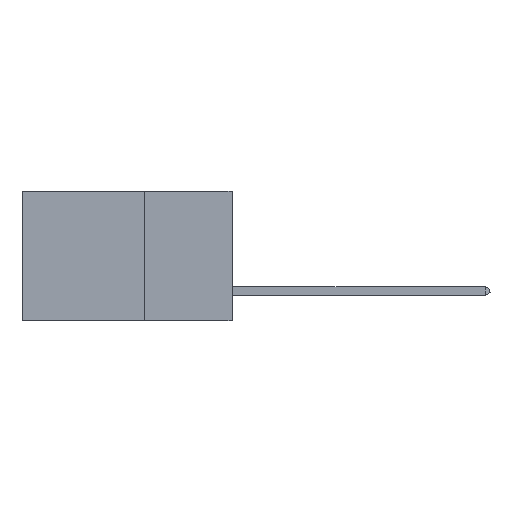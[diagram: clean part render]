
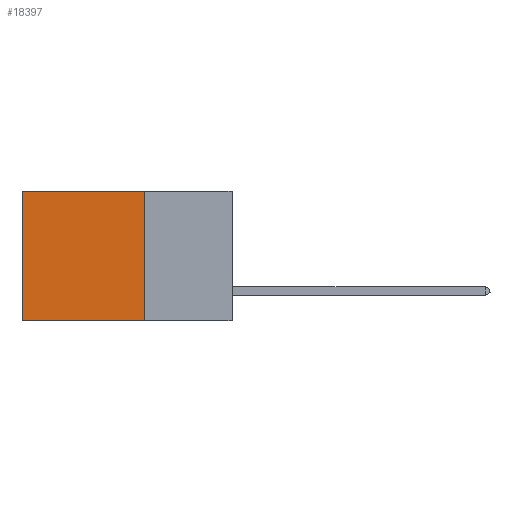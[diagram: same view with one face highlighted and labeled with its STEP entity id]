
A CAD part, left-side view. The second image highlights one B-rep face of the part: STEP entity #18397.
In plain terms, the highlighted planar face has unit normal (-1, 0, 0).
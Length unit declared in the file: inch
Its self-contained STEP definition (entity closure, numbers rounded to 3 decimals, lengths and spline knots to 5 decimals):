
#1252 = VECTOR ( 'NONE', #1528, 39.37008 ) ;
#1479 = VERTEX_POINT ( 'NONE', #2899 ) ;
#1528 = DIRECTION ( 'NONE',  ( 0., 0., -1. ) ) ;
#1542 = VERTEX_POINT ( 'NONE', #2821 ) ;
#2821 = CARTESIAN_POINT ( 'NONE',  ( 0.2875, 0.6, 0. ) ) ;
#2899 = CARTESIAN_POINT ( 'NONE',  ( 0.2875, 0.25, 0. ) ) ;
#3000 = EDGE_CURVE ( 'NONE', #1479, #17118, #3886, .T. ) ;
#3084 = EDGE_CURVE ( 'NONE', #1479, #1542, #9655, .T. ) ;
#3738 = ORIENTED_EDGE ( 'NONE', *, *, #3084, .T. ) ;
#3886 = LINE ( 'NONE', #14391, #18161 ) ;
#4565 = CARTESIAN_POINT ( 'NONE',  ( 0.2875, 0.25, -0.37 ) ) ;
#4890 = CARTESIAN_POINT ( 'NONE',  ( 0.2875, 0.25, -0.37 ) ) ;
#5632 = VECTOR ( 'NONE', #23377, 39.37008 ) ;
#6770 = CARTESIAN_POINT ( 'NONE',  ( 0.2875, 0.25, 0. ) ) ;
#6945 = CARTESIAN_POINT ( 'NONE',  ( 0.2875, 0.6, 0. ) ) ;
#6959 = AXIS2_PLACEMENT_3D ( 'NONE', #6770, #14138, #10630 ) ;
#7361 = EDGE_CURVE ( 'NONE', #17118, #18841, #10676, .T. ) ;
#9444 = FACE_OUTER_BOUND ( 'NONE', #11082, .T. ) ;
#9655 = LINE ( 'NONE', #16341, #5632 ) ;
#10630 = DIRECTION ( 'NONE',  ( 0., 0., -1. ) ) ;
#10676 = LINE ( 'NONE', #4565, #14798 ) ;
#10966 = CARTESIAN_POINT ( 'NONE',  ( 0.2875, 0.6, -0.37 ) ) ;
#11082 = EDGE_LOOP ( 'NONE', ( #17975, #22650, #11957, #3738 ) ) ;
#11957 = ORIENTED_EDGE ( 'NONE', *, *, #3000, .F. ) ;
#13404 = LINE ( 'NONE', #6945, #1252 ) ;
#14138 = DIRECTION ( 'NONE',  ( 1., 0., 0. ) ) ;
#14391 = CARTESIAN_POINT ( 'NONE',  ( 0.2875, 0.25, 0. ) ) ;
#14798 = VECTOR ( 'NONE', #20178, 39.37008 ) ;
#16341 = CARTESIAN_POINT ( 'NONE',  ( 0.2875, 0.25, 0. ) ) ;
#17118 = VERTEX_POINT ( 'NONE', #4890 ) ;
#17896 = PLANE ( 'NONE',  #6959 ) ;
#17975 = ORIENTED_EDGE ( 'NONE', *, *, #20357, .T. ) ;
#18161 = VECTOR ( 'NONE', #21415, 39.37008 ) ;
#18397 = ADVANCED_FACE ( 'NONE', ( #9444 ), #17896, .F. ) ;
#18841 = VERTEX_POINT ( 'NONE', #10966 ) ;
#20178 = DIRECTION ( 'NONE',  ( 0., 1., 0. ) ) ;
#20357 = EDGE_CURVE ( 'NONE', #1542, #18841, #13404, .T. ) ;
#21415 = DIRECTION ( 'NONE',  ( 0., 0., -1. ) ) ;
#22650 = ORIENTED_EDGE ( 'NONE', *, *, #7361, .F. ) ;
#23377 = DIRECTION ( 'NONE',  ( 0., 1., 0. ) ) ;
